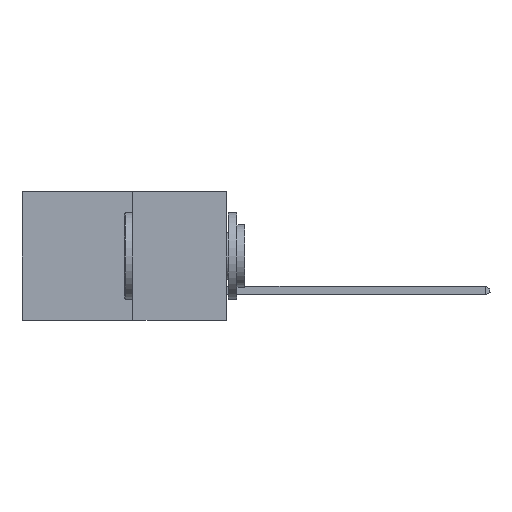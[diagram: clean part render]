
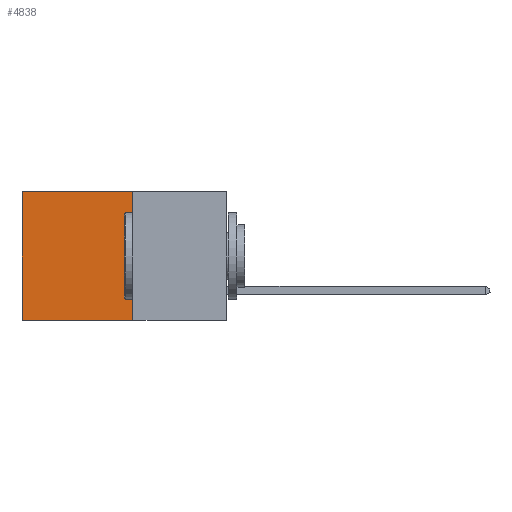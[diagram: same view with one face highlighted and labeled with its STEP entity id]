
A CAD part, left-side view. The second image highlights one B-rep face of the part: STEP entity #4838.
In plain terms, the highlighted planar face has unit normal (-1, 0, 0).
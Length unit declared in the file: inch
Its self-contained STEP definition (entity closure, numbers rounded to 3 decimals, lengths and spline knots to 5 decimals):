
#33 = AXIS2_PLACEMENT_3D ( 'NONE', #12547, #12298, #12276 ) ;
#114 = CARTESIAN_POINT ( 'NONE',  ( 0.277, 0.27, -0.37 ) ) ;
#616 = CARTESIAN_POINT ( 'NONE',  ( 0.277, 0.27, 0. ) ) ;
#1042 = EDGE_LOOP ( 'NONE', ( #20124, #7057, #6715, #18044 ) ) ;
#1381 = LINE ( 'NONE', #10389, #10255 ) ;
#1423 = LINE ( 'NONE', #616, #19486 ) ;
#1704 = EDGE_CURVE ( 'NONE', #10392, #18272, #1381, .T. ) ;
#2884 = EDGE_CURVE ( 'NONE', #18567, #12421, #22222, .T. ) ;
#3738 = DIRECTION ( 'NONE',  ( 0., 1., 0. ) ) ;
#4426 = CARTESIAN_POINT ( 'NONE',  ( 0.277, 0.27, -0.37 ) ) ;
#4838 = ADVANCED_FACE ( 'NONE', ( #13749 ), #13325, .F. ) ;
#6715 = ORIENTED_EDGE ( 'NONE', *, *, #1704, .F. ) ;
#7057 = ORIENTED_EDGE ( 'NONE', *, *, #21617, .F. ) ;
#8971 = VECTOR ( 'NONE', #11852, 39.37008 ) ;
#10255 = VECTOR ( 'NONE', #21398, 39.37008 ) ;
#10389 = CARTESIAN_POINT ( 'NONE',  ( 0.277, 0.27, -0.37 ) ) ;
#10392 = VERTEX_POINT ( 'NONE', #12491 ) ;
#11227 = CARTESIAN_POINT ( 'NONE',  ( 0.277, 0.59, -0.37 ) ) ;
#11852 = DIRECTION ( 'NONE',  ( 0., 0., -1. ) ) ;
#12276 = DIRECTION ( 'NONE',  ( 0., 0., -1. ) ) ;
#12298 = DIRECTION ( 'NONE',  ( 1., 0., 0. ) ) ;
#12421 = VERTEX_POINT ( 'NONE', #14647 ) ;
#12491 = CARTESIAN_POINT ( 'NONE',  ( 0.277, 0.27, 0. ) ) ;
#12547 = CARTESIAN_POINT ( 'NONE',  ( 0.277, 0.27, -0.37 ) ) ;
#13325 = PLANE ( 'NONE',  #33 ) ;
#13749 = FACE_OUTER_BOUND ( 'NONE', #1042, .T. ) ;
#14647 = CARTESIAN_POINT ( 'NONE',  ( 0.277, 0.59, -0.37 ) ) ;
#14681 = DIRECTION ( 'NONE',  ( 0., 1., 0. ) ) ;
#15527 = EDGE_CURVE ( 'NONE', #10392, #18567, #1423, .T. ) ;
#18044 = ORIENTED_EDGE ( 'NONE', *, *, #15527, .T. ) ;
#18272 = VERTEX_POINT ( 'NONE', #4426 ) ;
#18567 = VERTEX_POINT ( 'NONE', #22558 ) ;
#19486 = VECTOR ( 'NONE', #14681, 39.37008 ) ;
#20124 = ORIENTED_EDGE ( 'NONE', *, *, #2884, .T. ) ;
#20232 = VECTOR ( 'NONE', #3738, 39.37008 ) ;
#20756 = LINE ( 'NONE', #114, #20232 ) ;
#21398 = DIRECTION ( 'NONE',  ( 0., 0., -1. ) ) ;
#21617 = EDGE_CURVE ( 'NONE', #18272, #12421, #20756, .T. ) ;
#22222 = LINE ( 'NONE', #11227, #8971 ) ;
#22558 = CARTESIAN_POINT ( 'NONE',  ( 0.277, 0.59, 0. ) ) ;
